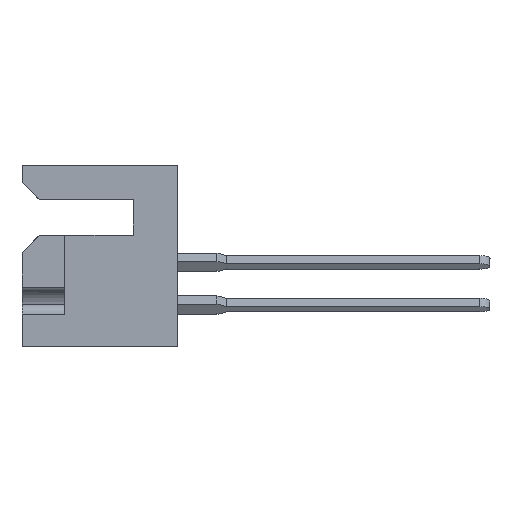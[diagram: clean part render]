
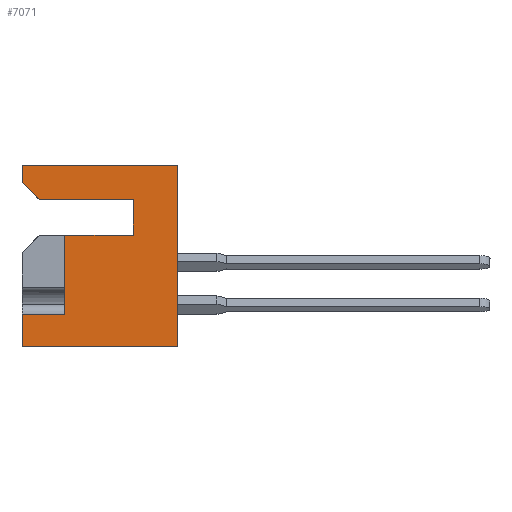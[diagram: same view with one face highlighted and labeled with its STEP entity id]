
A CAD part, left-side view. The second image highlights one B-rep face of the part: STEP entity #7071.
In plain terms, the highlighted planar face has unit normal (-1, 0, 0).
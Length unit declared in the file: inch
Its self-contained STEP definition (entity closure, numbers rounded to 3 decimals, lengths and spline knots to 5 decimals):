
#77 = VECTOR ( 'NONE', #8181, 39.37008 ) ;
#138 = DIRECTION ( 'NONE',  ( 0., -1., 0. ) ) ;
#140 = EDGE_CURVE ( 'NONE', #18275, #13186, #5855, .T. ) ;
#204 = DIRECTION ( 'NONE',  ( 0., 0., -1. ) ) ;
#658 = CARTESIAN_POINT ( 'NONE',  ( 0., 0.328, -0.205 ) ) ;
#701 = CARTESIAN_POINT ( 'NONE',  ( 0., 0.128, -0.1 ) ) ;
#721 = DIRECTION ( 'NONE',  ( 0., 0., 1. ) ) ;
#728 = VECTOR ( 'NONE', #721, 39.37008 ) ;
#794 = CARTESIAN_POINT ( 'NONE',  ( 0., 0.403, -0.1 ) ) ;
#1132 = ORIENTED_EDGE ( 'NONE', *, *, #13759, .T. ) ;
#1136 = LINE ( 'NONE', #14118, #10336 ) ;
#1506 = LINE ( 'NONE', #2259, #8300 ) ;
#1998 = LINE ( 'NONE', #14702, #6874 ) ;
#2259 = CARTESIAN_POINT ( 'NONE',  ( 0., 0.453, 0. ) ) ;
#2328 = VERTEX_POINT ( 'NONE', #13566 ) ;
#2812 = LINE ( 'NONE', #794, #14638 ) ;
#3828 = EDGE_CURVE ( 'NONE', #2328, #17106, #1506, .T. ) ;
#3962 = LINE ( 'NONE', #5553, #11694 ) ;
#4295 = CARTESIAN_POINT ( 'NONE',  ( 0., 0.328, -0.437 ) ) ;
#5125 = CARTESIAN_POINT ( 'NONE',  ( 0., 0.328, -0.205 ) ) ;
#5450 = ORIENTED_EDGE ( 'NONE', *, *, #19323, .T. ) ;
#5553 = CARTESIAN_POINT ( 'NONE',  ( 0., 0.128, -0.1 ) ) ;
#5855 = LINE ( 'NONE', #658, #728 ) ;
#6270 = AXIS2_PLACEMENT_3D ( 'NONE', #14193, #11116, #204 ) ;
#6751 = ORIENTED_EDGE ( 'NONE', *, *, #18236, .F. ) ;
#6758 = EDGE_CURVE ( 'NONE', #13725, #12451, #3962, .T. ) ;
#6874 = VECTOR ( 'NONE', #17797, 39.37008 ) ;
#6995 = FACE_OUTER_BOUND ( 'NONE', #11486, .T. ) ;
#7071 = ADVANCED_FACE ( 'NONE', ( #6995 ), #18727, .F. ) ;
#7142 = DIRECTION ( 'NONE',  ( 0., 0., 1. ) ) ;
#7342 = ORIENTED_EDGE ( 'NONE', *, *, #140, .F. ) ;
#7819 = DIRECTION ( 'NONE',  ( 0., 0., 1. ) ) ;
#7888 = CARTESIAN_POINT ( 'NONE',  ( 0., 0.128, -0.1 ) ) ;
#7961 = EDGE_CURVE ( 'NONE', #18352, #18418, #11991, .T. ) ;
#7963 = EDGE_CURVE ( 'NONE', #2328, #12451, #2812, .T. ) ;
#8145 = ORIENTED_EDGE ( 'NONE', *, *, #13809, .F. ) ;
#8181 = DIRECTION ( 'NONE',  ( 0., 0., 1. ) ) ;
#8300 = VECTOR ( 'NONE', #11583, 39.37008 ) ;
#8774 = CARTESIAN_POINT ( 'NONE',  ( 0., 0.453, 0. ) ) ;
#9008 = ORIENTED_EDGE ( 'NONE', *, *, #13510, .T. ) ;
#9786 = LINE ( 'NONE', #701, #77 ) ;
#10303 = CARTESIAN_POINT ( 'NONE',  ( 0., 0.328, -0.437 ) ) ;
#10336 = VECTOR ( 'NONE', #7819, 39.37008 ) ;
#10590 = CARTESIAN_POINT ( 'NONE',  ( 0., 0.453, -0.437 ) ) ;
#11116 = DIRECTION ( 'NONE',  ( 1., 0., 0. ) ) ;
#11465 = VERTEX_POINT ( 'NONE', #10590 ) ;
#11486 = EDGE_LOOP ( 'NONE', ( #9008, #6751, #16056, #1132, #8145, #15822, #14119, #13163, #15355, #5450, #7342 ) ) ;
#11583 = DIRECTION ( 'NONE',  ( 0., 0., 1. ) ) ;
#11694 = VECTOR ( 'NONE', #17779, 39.37008 ) ;
#11968 = LINE ( 'NONE', #8774, #19197 ) ;
#11991 = LINE ( 'NONE', #13289, #19221 ) ;
#12082 = CARTESIAN_POINT ( 'NONE',  ( 0., 0.403, -0.1 ) ) ;
#12164 = CARTESIAN_POINT ( 'NONE',  ( 0., 0.453, -0.531 ) ) ;
#12451 = VERTEX_POINT ( 'NONE', #12082 ) ;
#12516 = LINE ( 'NONE', #4295, #19961 ) ;
#12911 = VERTEX_POINT ( 'NONE', #19669 ) ;
#13163 = ORIENTED_EDGE ( 'NONE', *, *, #6758, .F. ) ;
#13186 = VERTEX_POINT ( 'NONE', #5125 ) ;
#13289 = CARTESIAN_POINT ( 'NONE',  ( 0., 0.453, -0.531 ) ) ;
#13347 = DIRECTION ( 'NONE',  ( 0., -0.707, -0.707 ) ) ;
#13510 = EDGE_CURVE ( 'NONE', #18275, #11465, #12516, .T. ) ;
#13566 = CARTESIAN_POINT ( 'NONE',  ( 0., 0.453, -0.05 ) ) ;
#13725 = VERTEX_POINT ( 'NONE', #7888 ) ;
#13759 = EDGE_CURVE ( 'NONE', #18418, #12911, #1136, .T. ) ;
#13809 = EDGE_CURVE ( 'NONE', #17106, #12911, #19714, .T. ) ;
#14118 = CARTESIAN_POINT ( 'NONE',  ( 0., 0., 0. ) ) ;
#14119 = ORIENTED_EDGE ( 'NONE', *, *, #7963, .T. ) ;
#14193 = CARTESIAN_POINT ( 'NONE',  ( 0., 0.453, 0. ) ) ;
#14638 = VECTOR ( 'NONE', #13347, 39.37008 ) ;
#14702 = CARTESIAN_POINT ( 'NONE',  ( 0., 0.128, -0.205 ) ) ;
#15355 = ORIENTED_EDGE ( 'NONE', *, *, #16156, .F. ) ;
#15822 = ORIENTED_EDGE ( 'NONE', *, *, #3828, .F. ) ;
#16056 = ORIENTED_EDGE ( 'NONE', *, *, #7961, .T. ) ;
#16156 = EDGE_CURVE ( 'NONE', #19123, #13725, #9786, .T. ) ;
#16669 = DIRECTION ( 'NONE',  ( 0., 1., 0. ) ) ;
#16935 = CARTESIAN_POINT ( 'NONE',  ( 0., 0.453, 0. ) ) ;
#17025 = CARTESIAN_POINT ( 'NONE',  ( 0., 0.453, 0. ) ) ;
#17072 = CARTESIAN_POINT ( 'NONE',  ( 0., 0.128, -0.205 ) ) ;
#17106 = VERTEX_POINT ( 'NONE', #16935 ) ;
#17551 = VECTOR ( 'NONE', #138, 39.37008 ) ;
#17779 = DIRECTION ( 'NONE',  ( 0., 1., 0. ) ) ;
#17797 = DIRECTION ( 'NONE',  ( 0., 1., 0. ) ) ;
#18010 = DIRECTION ( 'NONE',  ( 0., -1., 0. ) ) ;
#18236 = EDGE_CURVE ( 'NONE', #18352, #11465, #11968, .T. ) ;
#18275 = VERTEX_POINT ( 'NONE', #10303 ) ;
#18352 = VERTEX_POINT ( 'NONE', #12164 ) ;
#18418 = VERTEX_POINT ( 'NONE', #19564 ) ;
#18727 = PLANE ( 'NONE',  #6270 ) ;
#19123 = VERTEX_POINT ( 'NONE', #17072 ) ;
#19197 = VECTOR ( 'NONE', #7142, 39.37008 ) ;
#19221 = VECTOR ( 'NONE', #18010, 39.37008 ) ;
#19323 = EDGE_CURVE ( 'NONE', #19123, #13186, #1998, .T. ) ;
#19564 = CARTESIAN_POINT ( 'NONE',  ( 0., 0., -0.531 ) ) ;
#19669 = CARTESIAN_POINT ( 'NONE',  ( 0., 0., 0. ) ) ;
#19714 = LINE ( 'NONE', #17025, #17551 ) ;
#19961 = VECTOR ( 'NONE', #16669, 39.37008 ) ;
